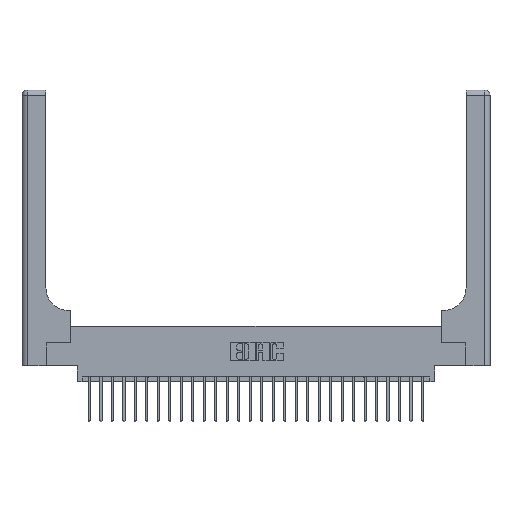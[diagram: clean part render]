
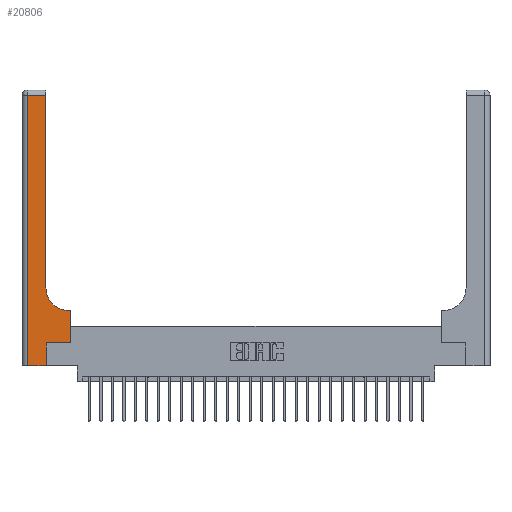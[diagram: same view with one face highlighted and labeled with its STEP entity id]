
A CAD part, top view. The second image highlights one B-rep face of the part: STEP entity #20806.
In plain terms, the highlighted planar face has unit normal (0, 0, 1).
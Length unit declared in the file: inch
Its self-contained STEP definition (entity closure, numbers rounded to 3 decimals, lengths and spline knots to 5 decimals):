
#253 = ORIENTED_EDGE ( 'NONE', *, *, #23038, .T. ) ;
#853 = CARTESIAN_POINT ( 'NONE',  ( 0.265, 0., 0.37 ) ) ;
#1194 = EDGE_LOOP ( 'NONE', ( #19861, #253, #11743, #17644, #7094, #21686, #5685, #20309, #19442 ) ) ;
#1594 = VERTEX_POINT ( 'NONE', #7778 ) ;
#2649 = CARTESIAN_POINT ( 'NONE',  ( 0.26, 2.94, 0.37 ) ) ;
#2813 = LINE ( 'NONE', #10997, #21407 ) ;
#3090 = VECTOR ( 'NONE', #18226, 39.37008 ) ;
#3275 = VERTEX_POINT ( 'NONE', #5970 ) ;
#3444 = CARTESIAN_POINT ( 'NONE',  ( 0.26, 0.85, 0.37 ) ) ;
#4164 = PLANE ( 'NONE',  #10193 ) ;
#4888 = EDGE_CURVE ( 'NONE', #22042, #24927, #2813, .T. ) ;
#4928 = EDGE_CURVE ( 'NONE', #24927, #21464, #5892, .T. ) ;
#4959 = CARTESIAN_POINT ( 'NONE',  ( 0.265, 0.25, 0.37 ) ) ;
#4999 = EDGE_CURVE ( 'NONE', #9177, #23496, #24194, .T. ) ;
#5220 = VERTEX_POINT ( 'NONE', #23638 ) ;
#5685 = ORIENTED_EDGE ( 'NONE', *, *, #13737, .T. ) ;
#5892 = LINE ( 'NONE', #18366, #13157 ) ;
#5970 = CARTESIAN_POINT ( 'NONE',  ( 0.528, 0.6, 0.37 ) ) ;
#7094 = ORIENTED_EDGE ( 'NONE', *, *, #8408, .T. ) ;
#7778 = CARTESIAN_POINT ( 'NONE',  ( 0.528, 0.25, 0.37 ) ) ;
#8216 = VERTEX_POINT ( 'NONE', #22547 ) ;
#8377 = DIRECTION ( 'NONE',  ( -1., 0., 0. ) ) ;
#8408 = EDGE_CURVE ( 'NONE', #21464, #5220, #15073, .T. ) ;
#9177 = VERTEX_POINT ( 'NONE', #3444 ) ;
#9410 = CIRCLE ( 'NONE', #19085, 0.25 ) ;
#10133 = DIRECTION ( 'NONE',  ( 0., 0., -1. ) ) ;
#10193 = AXIS2_PLACEMENT_3D ( 'NONE', #12511, #10133, #8377 ) ;
#10997 = CARTESIAN_POINT ( 'NONE',  ( 0.06, 3., 0.37 ) ) ;
#11473 = EDGE_CURVE ( 'NONE', #8216, #9177, #9410, .T. ) ;
#11743 = ORIENTED_EDGE ( 'NONE', *, *, #4888, .T. ) ;
#12242 = FACE_OUTER_BOUND ( 'NONE', #1194, .T. ) ;
#12511 = CARTESIAN_POINT ( 'NONE',  ( 0., 3., 0.37 ) ) ;
#12554 = CARTESIAN_POINT ( 'NONE',  ( 0.265, 0., 0.37 ) ) ;
#12809 = CARTESIAN_POINT ( 'NONE',  ( 0.06, 0., 0.37 ) ) ;
#13047 = VECTOR ( 'NONE', #18432, 39.37008 ) ;
#13157 = VECTOR ( 'NONE', #16438, 39.37008 ) ;
#13309 = DIRECTION ( 'NONE',  ( 1., 0., 0. ) ) ;
#13394 = VECTOR ( 'NONE', #20210, 39.37008 ) ;
#13737 = EDGE_CURVE ( 'NONE', #1594, #3275, #17239, .T. ) ;
#13867 = VECTOR ( 'NONE', #13309, 39.37008 ) ;
#15073 = LINE ( 'NONE', #853, #22934 ) ;
#16438 = DIRECTION ( 'NONE',  ( 1., 0., 0. ) ) ;
#17239 = LINE ( 'NONE', #25546, #18777 ) ;
#17644 = ORIENTED_EDGE ( 'NONE', *, *, #4928, .T. ) ;
#18226 = DIRECTION ( 'NONE',  ( 0., 1., 0. ) ) ;
#18297 = CARTESIAN_POINT ( 'NONE',  ( 0.26, 0.6, 0.37 ) ) ;
#18366 = CARTESIAN_POINT ( 'NONE',  ( 0., 0., 0.37 ) ) ;
#18432 = DIRECTION ( 'NONE',  ( -1., 0., 0. ) ) ;
#18694 = CARTESIAN_POINT ( 'NONE',  ( 0.06, 2.94, 0.37 ) ) ;
#18777 = VECTOR ( 'NONE', #21952, 39.37008 ) ;
#19085 = AXIS2_PLACEMENT_3D ( 'NONE', #19091, #23438, #21511 ) ;
#19091 = CARTESIAN_POINT ( 'NONE',  ( 0.51, 0.85, 0.37 ) ) ;
#19361 = DIRECTION ( 'NONE',  ( 0., -1., 0. ) ) ;
#19442 = ORIENTED_EDGE ( 'NONE', *, *, #11473, .T. ) ;
#19861 = ORIENTED_EDGE ( 'NONE', *, *, #4999, .T. ) ;
#20110 = CARTESIAN_POINT ( 'NONE',  ( 0.26, 3., 0.37 ) ) ;
#20210 = DIRECTION ( 'NONE',  ( -1., 0., 0. ) ) ;
#20309 = ORIENTED_EDGE ( 'NONE', *, *, #24783, .T. ) ;
#20806 = ADVANCED_FACE ( 'NONE', ( #12242 ), #4164, .F. ) ;
#21407 = VECTOR ( 'NONE', #19361, 39.37008 ) ;
#21464 = VERTEX_POINT ( 'NONE', #12554 ) ;
#21511 = DIRECTION ( 'NONE',  ( 1., 0., 0. ) ) ;
#21686 = ORIENTED_EDGE ( 'NONE', *, *, #23690, .T. ) ;
#21952 = DIRECTION ( 'NONE',  ( 0., 1., 0. ) ) ;
#22042 = VERTEX_POINT ( 'NONE', #18694 ) ;
#22348 = LINE ( 'NONE', #18297, #13047 ) ;
#22547 = CARTESIAN_POINT ( 'NONE',  ( 0.51, 0.6, 0.37 ) ) ;
#22934 = VECTOR ( 'NONE', #23384, 39.37008 ) ;
#23038 = EDGE_CURVE ( 'NONE', #23496, #22042, #24431, .T. ) ;
#23384 = DIRECTION ( 'NONE',  ( 0., 1., 0. ) ) ;
#23438 = DIRECTION ( 'NONE',  ( 0., 0., -1. ) ) ;
#23496 = VERTEX_POINT ( 'NONE', #2649 ) ;
#23638 = CARTESIAN_POINT ( 'NONE',  ( 0.265, 0.25, 0.37 ) ) ;
#23666 = LINE ( 'NONE', #4959, #13867 ) ;
#23690 = EDGE_CURVE ( 'NONE', #5220, #1594, #23666, .T. ) ;
#24194 = LINE ( 'NONE', #20110, #3090 ) ;
#24431 = LINE ( 'NONE', #26751, #13394 ) ;
#24783 = EDGE_CURVE ( 'NONE', #3275, #8216, #22348, .T. ) ;
#24927 = VERTEX_POINT ( 'NONE', #12809 ) ;
#25546 = CARTESIAN_POINT ( 'NONE',  ( 0.528, 0.25, 0.37 ) ) ;
#26751 = CARTESIAN_POINT ( 'NONE',  ( 0., 2.94, 0.37 ) ) ;
